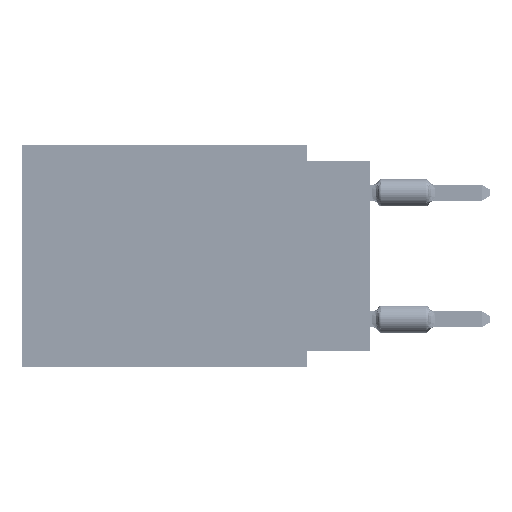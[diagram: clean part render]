
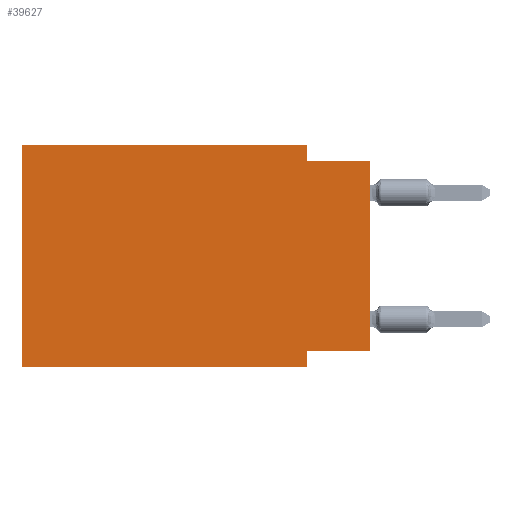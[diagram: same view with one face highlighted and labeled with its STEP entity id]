
A CAD part, left-side view. The second image highlights one B-rep face of the part: STEP entity #39627.
In plain terms, the highlighted planar face has unit normal (-1, 0, 0).
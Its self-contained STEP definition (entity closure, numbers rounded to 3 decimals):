
#433 = VECTOR ( 'NONE', #24247, 1000. ) ;
#759 = VERTEX_POINT ( 'NONE', #11903 ) ;
#797 = VECTOR ( 'NONE', #57473, 1000. ) ;
#2357 = AXIS2_PLACEMENT_3D ( 'NONE', #108519, #73068, #54472 ) ;
#3863 = ORIENTED_EDGE ( 'NONE', *, *, #40440, .F. ) ;
#4098 = CARTESIAN_POINT ( 'NONE',  ( 0., 13.97, 0. ) ) ;
#4328 = CARTESIAN_POINT ( 'NONE',  ( 0., 13.97, -8.89 ) ) ;
#4680 = DIRECTION ( 'NONE',  ( 0., 0., 1. ) ) ;
#5674 = VECTOR ( 'NONE', #25892, 1000. ) ;
#6096 = DIRECTION ( 'NONE',  ( 0., -1., 0. ) ) ;
#6365 = CARTESIAN_POINT ( 'NONE',  ( 0., 2.54, 0. ) ) ;
#6476 = ORIENTED_EDGE ( 'NONE', *, *, #116116, .F. ) ;
#7552 = LINE ( 'NONE', #6365, #79113 ) ;
#10097 = CARTESIAN_POINT ( 'NONE',  ( 0., 0., -0.635 ) ) ;
#11903 = CARTESIAN_POINT ( 'NONE',  ( 0., 0., -0.635 ) ) ;
#12848 = VERTEX_POINT ( 'NONE', #103545 ) ;
#13187 = ORIENTED_EDGE ( 'NONE', *, *, #43709, .F. ) ;
#16406 = ORIENTED_EDGE ( 'NONE', *, *, #82593, .F. ) ;
#17997 = ORIENTED_EDGE ( 'NONE', *, *, #49846, .F. ) ;
#20874 = LINE ( 'NONE', #10097, #797 ) ;
#22171 = CARTESIAN_POINT ( 'NONE',  ( 0., 0., -8.255 ) ) ;
#22704 = EDGE_CURVE ( 'NONE', #68321, #59492, #57515, .T. ) ;
#23175 = VECTOR ( 'NONE', #6096, 1000. ) ;
#24247 = DIRECTION ( 'NONE',  ( 0., -1., 0. ) ) ;
#24954 = ORIENTED_EDGE ( 'NONE', *, *, #109540, .T. ) ;
#25647 = VECTOR ( 'NONE', #58772, 1000. ) ;
#25892 = DIRECTION ( 'NONE',  ( 0., 0., -1. ) ) ;
#31098 = ORIENTED_EDGE ( 'NONE', *, *, #22704, .F. ) ;
#36459 = VERTEX_POINT ( 'NONE', #112965 ) ;
#37030 = CARTESIAN_POINT ( 'NONE',  ( 0., 13.97, 0. ) ) ;
#39627 = ADVANCED_FACE ( 'NONE', ( #71322 ), #45450, .F. ) ;
#40440 = EDGE_CURVE ( 'NONE', #59492, #62978, #69255, .T. ) ;
#43352 = CARTESIAN_POINT ( 'NONE',  ( 0., 13.97, -8.89 ) ) ;
#43709 = EDGE_CURVE ( 'NONE', #62978, #36459, #7552, .T. ) ;
#43823 = CARTESIAN_POINT ( 'NONE',  ( 0., 0., 0. ) ) ;
#45450 = PLANE ( 'NONE',  #2357 ) ;
#46827 = LINE ( 'NONE', #83460, #5674 ) ;
#49846 = EDGE_CURVE ( 'NONE', #101308, #12848, #46827, .T. ) ;
#50484 = CARTESIAN_POINT ( 'NONE',  ( 0., 2.54, 0. ) ) ;
#50509 = LINE ( 'NONE', #4328, #23175 ) ;
#50940 = LINE ( 'NONE', #22171, #25647 ) ;
#51321 = EDGE_CURVE ( 'NONE', #68321, #12848, #50509, .T. ) ;
#52691 = VECTOR ( 'NONE', #4680, 1000. ) ;
#54295 = EDGE_LOOP ( 'NONE', ( #24954, #16406, #13187, #3863, #31098, #69787, #17997, #6476 ) ) ;
#54472 = DIRECTION ( 'NONE',  ( 0., 0., -1. ) ) ;
#57473 = DIRECTION ( 'NONE',  ( 0., -1., 0. ) ) ;
#57515 = LINE ( 'NONE', #4098, #52691 ) ;
#58772 = DIRECTION ( 'NONE',  ( 0., 1., 0. ) ) ;
#59492 = VERTEX_POINT ( 'NONE', #37030 ) ;
#62733 = DIRECTION ( 'NONE',  ( 0., 0., -1. ) ) ;
#62978 = VERTEX_POINT ( 'NONE', #50484 ) ;
#68321 = VERTEX_POINT ( 'NONE', #43352 ) ;
#69255 = LINE ( 'NONE', #106457, #433 ) ;
#69787 = ORIENTED_EDGE ( 'NONE', *, *, #51321, .T. ) ;
#71322 = FACE_OUTER_BOUND ( 'NONE', #54295, .T. ) ;
#73068 = DIRECTION ( 'NONE',  ( 1., 0., 0. ) ) ;
#73382 = CARTESIAN_POINT ( 'NONE',  ( 0., 2.54, -8.255 ) ) ;
#79113 = VECTOR ( 'NONE', #62733, 1000. ) ;
#82120 = VECTOR ( 'NONE', #109208, 1000. ) ;
#82593 = EDGE_CURVE ( 'NONE', #36459, #759, #20874, .T. ) ;
#83460 = CARTESIAN_POINT ( 'NONE',  ( 0., 2.54, -8.89 ) ) ;
#93996 = VERTEX_POINT ( 'NONE', #105886 ) ;
#98461 = LINE ( 'NONE', #43823, #82120 ) ;
#101308 = VERTEX_POINT ( 'NONE', #73382 ) ;
#103545 = CARTESIAN_POINT ( 'NONE',  ( 0., 2.54, -8.89 ) ) ;
#105886 = CARTESIAN_POINT ( 'NONE',  ( 0., 0., -8.255 ) ) ;
#106457 = CARTESIAN_POINT ( 'NONE',  ( 0., 13.97, 0. ) ) ;
#108519 = CARTESIAN_POINT ( 'NONE',  ( 0., 13.97, 0. ) ) ;
#109208 = DIRECTION ( 'NONE',  ( 0., 0., 1. ) ) ;
#109540 = EDGE_CURVE ( 'NONE', #93996, #759, #98461, .T. ) ;
#112965 = CARTESIAN_POINT ( 'NONE',  ( 0., 2.54, -0.635 ) ) ;
#116116 = EDGE_CURVE ( 'NONE', #93996, #101308, #50940, .T. ) ;
